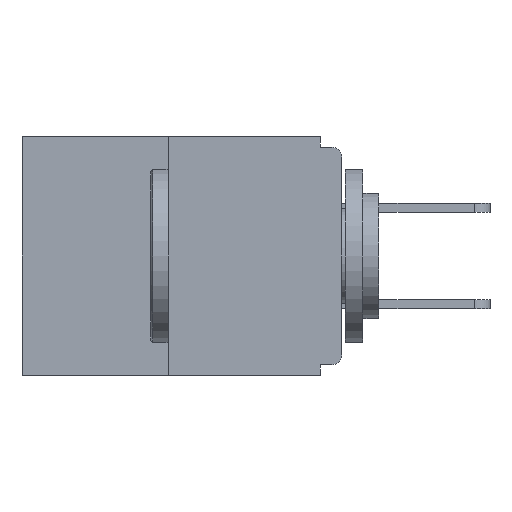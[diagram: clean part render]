
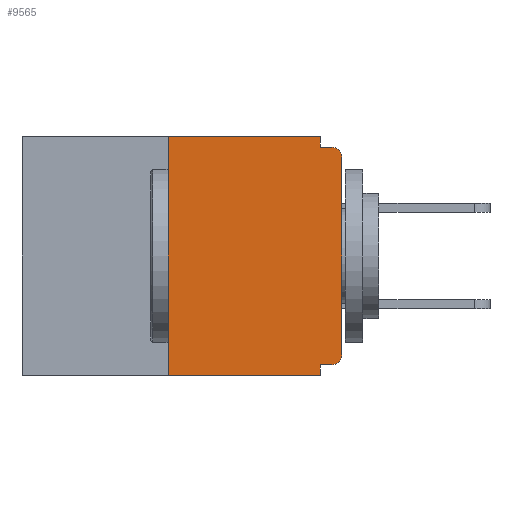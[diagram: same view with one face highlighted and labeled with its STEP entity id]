
A CAD part, left-side view. The second image highlights one B-rep face of the part: STEP entity #9565.
In plain terms, the highlighted planar face has unit normal (-1, 0, 0).
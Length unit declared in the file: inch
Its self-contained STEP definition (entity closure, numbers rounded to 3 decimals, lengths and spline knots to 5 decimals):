
#275 = CARTESIAN_POINT ( 'NONE',  ( 0., 0.031, -0.343 ) ) ;
#514 = VERTEX_POINT ( 'NONE', #7495 ) ;
#556 = DIRECTION ( 'NONE',  ( 0., 0., -1. ) ) ;
#1257 = DIRECTION ( 'NONE',  ( 0., 0., 1. ) ) ;
#2224 = CIRCLE ( 'NONE', #2977, 0.015 ) ;
#2454 = EDGE_CURVE ( 'NONE', #6787, #8156, #13295, .T. ) ;
#2528 = CARTESIAN_POINT ( 'NONE',  ( 0., 0.25, -0.343 ) ) ;
#2734 = ORIENTED_EDGE ( 'NONE', *, *, #10768, .T. ) ;
#2939 = EDGE_CURVE ( 'NONE', #13018, #14974, #2224, .T. ) ;
#2977 = AXIS2_PLACEMENT_3D ( 'NONE', #9788, #11510, #17190 ) ;
#3169 = EDGE_CURVE ( 'NONE', #14252, #14974, #19803, .T. ) ;
#3322 = VECTOR ( 'NONE', #4026, 39.37008 ) ;
#3355 = CARTESIAN_POINT ( 'NONE',  ( 0., 0.031, -0.343 ) ) ;
#3407 = ORIENTED_EDGE ( 'NONE', *, *, #21670, .T. ) ;
#3751 = AXIS2_PLACEMENT_3D ( 'NONE', #9216, #19441, #5796 ) ;
#4026 = DIRECTION ( 'NONE',  ( 0., 0., 1. ) ) ;
#4179 = CARTESIAN_POINT ( 'NONE',  ( 0., 0., 0. ) ) ;
#4338 = EDGE_CURVE ( 'NONE', #17779, #5207, #21329, .T. ) ;
#4721 = EDGE_LOOP ( 'NONE', ( #8395, #14046, #19725, #15172, #15565, #2734, #3407, #21181, #16550, #6292 ) ) ;
#5207 = VERTEX_POINT ( 'NONE', #3355 ) ;
#5796 = DIRECTION ( 'NONE',  ( 0., 0., -1. ) ) ;
#5840 = DIRECTION ( 'NONE',  ( 0., -1., 0. ) ) ;
#6292 = ORIENTED_EDGE ( 'NONE', *, *, #21827, .F. ) ;
#6705 = CARTESIAN_POINT ( 'NONE',  ( 0., 0.031, -0.328 ) ) ;
#6712 = LINE ( 'NONE', #13217, #8619 ) ;
#6787 = VERTEX_POINT ( 'NONE', #10770 ) ;
#7278 = VECTOR ( 'NONE', #8893, 39.37008 ) ;
#7358 = VECTOR ( 'NONE', #21628, 39.37008 ) ;
#7469 = CARTESIAN_POINT ( 'NONE',  ( 0., 0., -0.328 ) ) ;
#7495 = CARTESIAN_POINT ( 'NONE',  ( 0., 0.015, -0.328 ) ) ;
#8079 = VERTEX_POINT ( 'NONE', #6705 ) ;
#8156 = VERTEX_POINT ( 'NONE', #8613 ) ;
#8395 = ORIENTED_EDGE ( 'NONE', *, *, #2454, .F. ) ;
#8509 = VECTOR ( 'NONE', #18059, 39.37008 ) ;
#8613 = CARTESIAN_POINT ( 'NONE',  ( 0., 0.031, 0. ) ) ;
#8619 = VECTOR ( 'NONE', #1257, 39.37008 ) ;
#8893 = DIRECTION ( 'NONE',  ( 0., 0., -1. ) ) ;
#8998 = PLANE ( 'NONE',  #3751 ) ;
#9200 = CARTESIAN_POINT ( 'NONE',  ( 0., 0.015, -0.015 ) ) ;
#9216 = CARTESIAN_POINT ( 'NONE',  ( 0., 0.46, 0. ) ) ;
#9227 = VECTOR ( 'NONE', #11114, 39.37008 ) ;
#9488 = CARTESIAN_POINT ( 'NONE',  ( 0., 0.46, -0.343 ) ) ;
#9565 = ADVANCED_FACE ( 'NONE', ( #20285 ), #8998, .F. ) ;
#9788 = CARTESIAN_POINT ( 'NONE',  ( 0., 0.015, -0.03 ) ) ;
#10281 = LINE ( 'NONE', #275, #7278 ) ;
#10768 = EDGE_CURVE ( 'NONE', #514, #16850, #13101, .T. ) ;
#10770 = CARTESIAN_POINT ( 'NONE',  ( 0., 0.25, 0. ) ) ;
#10814 = EDGE_CURVE ( 'NONE', #514, #8079, #15808, .T. ) ;
#11114 = DIRECTION ( 'NONE',  ( 0., -1., 0. ) ) ;
#11510 = DIRECTION ( 'NONE',  ( -1., 0., 0. ) ) ;
#12077 = VECTOR ( 'NONE', #5840, 39.37008 ) ;
#12391 = CARTESIAN_POINT ( 'NONE',  ( 0., 0., -0.313 ) ) ;
#12684 = CARTESIAN_POINT ( 'NONE',  ( 0., 0.015, -0.313 ) ) ;
#13018 = VERTEX_POINT ( 'NONE', #14278 ) ;
#13101 = CIRCLE ( 'NONE', #19169, 0.015 ) ;
#13217 = CARTESIAN_POINT ( 'NONE',  ( 0., 0.25, 0. ) ) ;
#13295 = LINE ( 'NONE', #16353, #7358 ) ;
#14046 = ORIENTED_EDGE ( 'NONE', *, *, #17819, .F. ) ;
#14155 = EDGE_CURVE ( 'NONE', #8079, #5207, #10281, .T. ) ;
#14187 = CARTESIAN_POINT ( 'NONE',  ( 0., 0.031, -0.015 ) ) ;
#14252 = VERTEX_POINT ( 'NONE', #14187 ) ;
#14278 = CARTESIAN_POINT ( 'NONE',  ( 0., 0., -0.03 ) ) ;
#14974 = VERTEX_POINT ( 'NONE', #9200 ) ;
#15172 = ORIENTED_EDGE ( 'NONE', *, *, #14155, .F. ) ;
#15565 = ORIENTED_EDGE ( 'NONE', *, *, #10814, .F. ) ;
#15808 = LINE ( 'NONE', #7469, #8509 ) ;
#16353 = CARTESIAN_POINT ( 'NONE',  ( 0., 0.46, 0. ) ) ;
#16550 = ORIENTED_EDGE ( 'NONE', *, *, #3169, .F. ) ;
#16850 = VERTEX_POINT ( 'NONE', #12391 ) ;
#17190 = DIRECTION ( 'NONE',  ( 0., 0., -1. ) ) ;
#17779 = VERTEX_POINT ( 'NONE', #2528 ) ;
#17819 = EDGE_CURVE ( 'NONE', #17779, #6787, #6712, .T. ) ;
#17991 = DIRECTION ( 'NONE',  ( -1., 0., 0. ) ) ;
#18059 = DIRECTION ( 'NONE',  ( 0., 1., 0. ) ) ;
#18444 = LINE ( 'NONE', #4179, #3322 ) ;
#18985 = VECTOR ( 'NONE', #556, 39.37008 ) ;
#19169 = AXIS2_PLACEMENT_3D ( 'NONE', #12684, #17991, #19744 ) ;
#19441 = DIRECTION ( 'NONE',  ( 1., 0., 0. ) ) ;
#19725 = ORIENTED_EDGE ( 'NONE', *, *, #4338, .T. ) ;
#19744 = DIRECTION ( 'NONE',  ( 0., 0., -1. ) ) ;
#19795 = CARTESIAN_POINT ( 'NONE',  ( 0., 0.031, 0. ) ) ;
#19803 = LINE ( 'NONE', #19987, #9227 ) ;
#19987 = CARTESIAN_POINT ( 'NONE',  ( 0., 0., -0.015 ) ) ;
#20285 = FACE_OUTER_BOUND ( 'NONE', #4721, .T. ) ;
#21181 = ORIENTED_EDGE ( 'NONE', *, *, #2939, .T. ) ;
#21329 = LINE ( 'NONE', #9488, #12077 ) ;
#21628 = DIRECTION ( 'NONE',  ( 0., -1., 0. ) ) ;
#21670 = EDGE_CURVE ( 'NONE', #16850, #13018, #18444, .T. ) ;
#21827 = EDGE_CURVE ( 'NONE', #8156, #14252, #22017, .T. ) ;
#22017 = LINE ( 'NONE', #19795, #18985 ) ;
